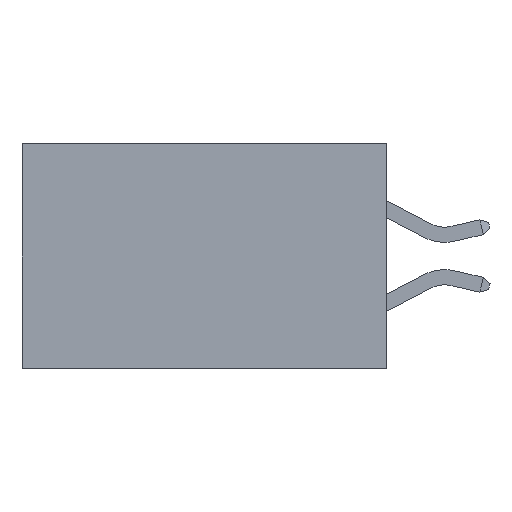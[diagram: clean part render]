
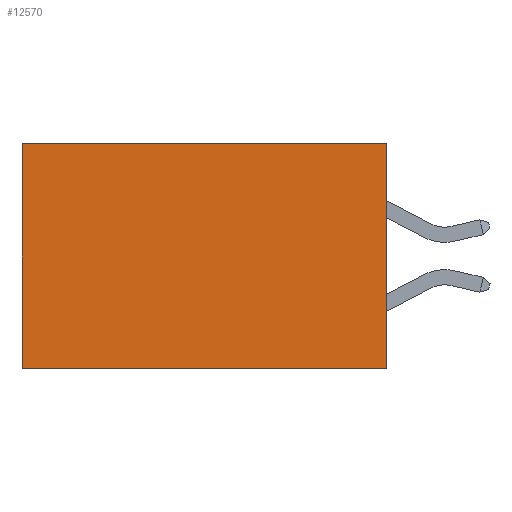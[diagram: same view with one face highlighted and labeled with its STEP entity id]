
A CAD part, left-side view. The second image highlights one B-rep face of the part: STEP entity #12570.
In plain terms, the highlighted planar face has unit normal (-1, 0, 0).
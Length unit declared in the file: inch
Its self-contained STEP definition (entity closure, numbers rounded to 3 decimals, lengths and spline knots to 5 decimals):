
#1105 = VERTEX_POINT ( 'NONE', #17248 ) ;
#1125 = EDGE_LOOP ( 'NONE', ( #6741, #10683, #16153, #14706 ) ) ;
#1680 = VECTOR ( 'NONE', #10520, 39.37008 ) ;
#2189 = LINE ( 'NONE', #18237, #1680 ) ;
#3037 = VERTEX_POINT ( 'NONE', #6130 ) ;
#4429 = CARTESIAN_POINT ( 'NONE',  ( 0.2615, 0., -0.37 ) ) ;
#4613 = EDGE_CURVE ( 'NONE', #8762, #1105, #9826, .T. ) ;
#4876 = CARTESIAN_POINT ( 'NONE',  ( 0.2615, 0., 0. ) ) ;
#5859 = VECTOR ( 'NONE', #10397, 39.37008 ) ;
#6130 = CARTESIAN_POINT ( 'NONE',  ( 0.2615, 0., 0. ) ) ;
#6346 = LINE ( 'NONE', #8818, #5859 ) ;
#6741 = ORIENTED_EDGE ( 'NONE', *, *, #4613, .T. ) ;
#7636 = DIRECTION ( 'NONE',  ( 0., 0., -1. ) ) ;
#7682 = EDGE_CURVE ( 'NONE', #3037, #8762, #13458, .T. ) ;
#7747 = CARTESIAN_POINT ( 'NONE',  ( 0.2615, 0.6, -0.37 ) ) ;
#8762 = VERTEX_POINT ( 'NONE', #19280 ) ;
#8818 = CARTESIAN_POINT ( 'NONE',  ( 0.2615, 0., -0.37 ) ) ;
#8925 = DIRECTION ( 'NONE',  ( 0., 0., -1. ) ) ;
#9545 = VERTEX_POINT ( 'NONE', #10207 ) ;
#9826 = LINE ( 'NONE', #7747, #17582 ) ;
#10207 = CARTESIAN_POINT ( 'NONE',  ( 0.2615, 0., -0.37 ) ) ;
#10342 = EDGE_CURVE ( 'NONE', #9545, #1105, #2189, .T. ) ;
#10397 = DIRECTION ( 'NONE',  ( 0., 0., -1. ) ) ;
#10520 = DIRECTION ( 'NONE',  ( 0., 1., 0. ) ) ;
#10683 = ORIENTED_EDGE ( 'NONE', *, *, #10342, .F. ) ;
#11188 = AXIS2_PLACEMENT_3D ( 'NONE', #4429, #16972, #7636 ) ;
#12570 = ADVANCED_FACE ( 'NONE', ( #15890 ), #19973, .F. ) ;
#12755 = DIRECTION ( 'NONE',  ( 0., 1., 0. ) ) ;
#13458 = LINE ( 'NONE', #4876, #18024 ) ;
#14706 = ORIENTED_EDGE ( 'NONE', *, *, #7682, .T. ) ;
#15890 = FACE_OUTER_BOUND ( 'NONE', #1125, .T. ) ;
#16153 = ORIENTED_EDGE ( 'NONE', *, *, #16475, .F. ) ;
#16475 = EDGE_CURVE ( 'NONE', #3037, #9545, #6346, .T. ) ;
#16972 = DIRECTION ( 'NONE',  ( 1., 0., 0. ) ) ;
#17248 = CARTESIAN_POINT ( 'NONE',  ( 0.2615, 0.6, -0.37 ) ) ;
#17582 = VECTOR ( 'NONE', #8925, 39.37008 ) ;
#18024 = VECTOR ( 'NONE', #12755, 39.37008 ) ;
#18237 = CARTESIAN_POINT ( 'NONE',  ( 0.2615, 0., -0.37 ) ) ;
#19280 = CARTESIAN_POINT ( 'NONE',  ( 0.2615, 0.6, 0. ) ) ;
#19973 = PLANE ( 'NONE',  #11188 ) ;
